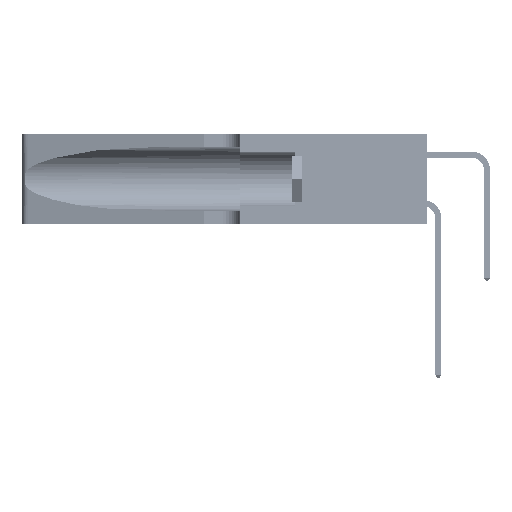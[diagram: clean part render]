
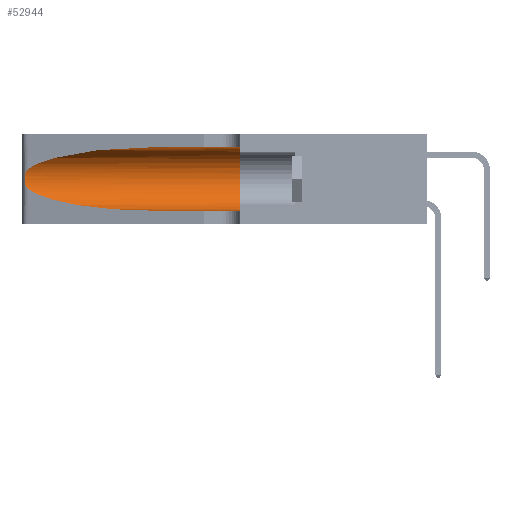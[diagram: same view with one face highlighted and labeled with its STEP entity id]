
A CAD part, left-side view. The second image highlights one B-rep face of the part: STEP entity #52944.
In plain terms, the highlighted cylindrical face has radius 3.308 mm (diameter 6.617 mm), a partial arc.
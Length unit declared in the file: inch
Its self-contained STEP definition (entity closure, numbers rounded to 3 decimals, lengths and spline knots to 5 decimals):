
#1289 = EDGE_CURVE ( 'NONE', #24550, #24707, #36671, .T. ) ;
#2194 = CARTESIAN_POINT ( 'NONE',  ( 0.26018, 1.23835, 0.19895 ) ) ;
#3975 = CARTESIAN_POINT ( 'NONE',  ( 0.18966, 0.96281, 0.31525 ) ) ;
#4296 = AXIS2_PLACEMENT_3D ( 'NONE', #30012, #25884, #5405 ) ;
#5024 = VERTEX_POINT ( 'NONE', #26585 ) ;
#5405 = DIRECTION ( 'NONE',  ( 0., 0., -1. ) ) ;
#6168 = CARTESIAN_POINT ( 'NONE',  ( 0.25555, 1.22994, 0.2215 ) ) ;
#6346 = CARTESIAN_POINT ( 'NONE',  ( 0.26075, 1.23896, 0.178 ) ) ;
#6778 = CARTESIAN_POINT ( 'NONE',  ( 0.1305, 1.61858, 0.31525 ) ) ;
#7345 = CARTESIAN_POINT ( 'NONE',  ( 0.18966, 0.96281, 0.05475 ) ) ;
#8405 = FACE_OUTER_BOUND ( 'NONE', #52028, .T. ) ;
#8641 = DIRECTION ( 'NONE',  ( 0., 1., 0. ) ) ;
#9437 = LINE ( 'NONE', #6778, #40942 ) ;
#9640 =( BOUNDED_CURVE ( )  B_SPLINE_CURVE ( 3, ( #27853, #52443, #7345, #36134 ),
 .UNSPECIFIED., .F., .T. ) 
 B_SPLINE_CURVE_WITH_KNOTS ( ( 4, 4 ),
 ( 3.44316, 4.71239 ),
 .UNSPECIFIED. ) 
 CURVE ( )  GEOMETRIC_REPRESENTATION_ITEM ( )  RATIONAL_B_SPLINE_CURVE ( ( 1., 0.87, 0.87, 1. ) ) 
 REPRESENTATION_ITEM ( '' )  );
#10225 = EDGE_CURVE ( 'NONE', #5024, #24550, #17521, .T. ) ;
#10495 = CARTESIAN_POINT ( 'NONE',  ( 0.25856, 1.23593, 0.16098 ) ) ;
#12281 = AXIS2_PLACEMENT_3D ( 'NONE', #33267, #8641, #37419 ) ;
#14595 = CARTESIAN_POINT ( 'NONE',  ( 0.25639, 1.23186, 0.15144 ) ) ;
#16179 = CIRCLE ( 'NONE', #12281, 0.13025 ) ;
#16218 = ORIENTED_EDGE ( 'NONE', *, *, #10225, .T. ) ;
#17521 =( BOUNDED_CURVE ( )  B_SPLINE_CURVE ( 3, ( #32737, #3975, #45147, #20523 ),
 .UNSPECIFIED., .F., .F. ) 
 B_SPLINE_CURVE_WITH_KNOTS ( ( 4, 4 ),
 ( 1.5708, 2.84003 ),
 .UNSPECIFIED. ) 
 CURVE ( )  GEOMETRIC_REPRESENTATION_ITEM ( )  RATIONAL_B_SPLINE_CURVE ( ( 1., 0.87, 0.87, 1. ) ) 
 REPRESENTATION_ITEM ( '' )  );
#17752 = CARTESIAN_POINT ( 'NONE',  ( 0.1305, 1.61858, 0.05475 ) ) ;
#18563 = CARTESIAN_POINT ( 'NONE',  ( 0.25639, 1.23184, 0.21858 ) ) ;
#18736 = CARTESIAN_POINT ( 'NONE',  ( 0.25487, 1.22718, 0.14631 ) ) ;
#20523 = CARTESIAN_POINT ( 'NONE',  ( 0.25487, 1.22718, 0.22369 ) ) ;
#20893 = CARTESIAN_POINT ( 'NONE',  ( 0.1305, 0.72297, 0.05475 ) ) ;
#22717 = CARTESIAN_POINT ( 'NONE',  ( 0.25487, 1.22718, 0.22369 ) ) ;
#24550 = VERTEX_POINT ( 'NONE', #39473 ) ;
#24707 = VERTEX_POINT ( 'NONE', #36575 ) ;
#24864 = VERTEX_POINT ( 'NONE', #20893 ) ;
#24978 = ORIENTED_EDGE ( 'NONE', *, *, #32246, .T. ) ;
#25884 = DIRECTION ( 'NONE',  ( 0., -1., 0. ) ) ;
#26585 = CARTESIAN_POINT ( 'NONE',  ( 0.1305, 0.72297, 0.31525 ) ) ;
#26829 = CARTESIAN_POINT ( 'NONE',  ( 0.25854, 1.2359, 0.20912 ) ) ;
#27078 = VECTOR ( 'NONE', #34307, 39.37008 ) ;
#27853 = CARTESIAN_POINT ( 'NONE',  ( 0.25487, 1.22718, 0.14631 ) ) ;
#27951 = CARTESIAN_POINT ( 'NONE',  ( 0.1305, 0.35, 0.05475 ) ) ;
#30012 = CARTESIAN_POINT ( 'NONE',  ( 0.1305, 1.61858, 0.185 ) ) ;
#30969 = CARTESIAN_POINT ( 'NONE',  ( 0.26075, 1.23896, 0.19203 ) ) ;
#31583 = ORIENTED_EDGE ( 'NONE', *, *, #1289, .T. ) ;
#32246 = EDGE_CURVE ( 'NONE', #24864, #35520, #40583, .T. ) ;
#32737 = CARTESIAN_POINT ( 'NONE',  ( 0.1305, 0.72297, 0.31525 ) ) ;
#33267 = CARTESIAN_POINT ( 'NONE',  ( 0.1305, 0.35, 0.185 ) ) ;
#34307 = DIRECTION ( 'NONE',  ( 0., -1., 0. ) ) ;
#35114 = CARTESIAN_POINT ( 'NONE',  ( 0.26017, 1.23833, 0.17102 ) ) ;
#35520 = VERTEX_POINT ( 'NONE', #27951 ) ;
#35771 = ORIENTED_EDGE ( 'NONE', *, *, #41002, .F. ) ;
#36134 = CARTESIAN_POINT ( 'NONE',  ( 0.1305, 0.72297, 0.05475 ) ) ;
#36146 = VERTEX_POINT ( 'NONE', #44068 ) ;
#36575 = CARTESIAN_POINT ( 'NONE',  ( 0.25487, 1.22718, 0.14631 ) ) ;
#36671 = B_SPLINE_CURVE_WITH_KNOTS ( 'NONE', 3,
 ( #22717, #6168, #18563, #51428, #26829, #2194, #30969, #6346, #35114, #10495, #39238, #14595, #43368, #18736 ),
 .UNSPECIFIED., .F., .F.,
 ( 4, 2, 2, 2, 2, 2, 4 ),
 ( 0., 0.00027, 0.00053, 0.00107, 0.0016, 0.00187, 0.00214 ),
 .UNSPECIFIED. ) ;
#37236 = ORIENTED_EDGE ( 'NONE', *, *, #38082, .T. ) ;
#37419 = DIRECTION ( 'NONE',  ( 0., 0., 1. ) ) ;
#38082 = EDGE_CURVE ( 'NONE', #24707, #24864, #9640, .T. ) ;
#39238 = CARTESIAN_POINT ( 'NONE',  ( 0.25789, 1.23486, 0.15765 ) ) ;
#39473 = CARTESIAN_POINT ( 'NONE',  ( 0.25487, 1.22718, 0.22369 ) ) ;
#39945 = CYLINDRICAL_SURFACE ( 'NONE', #4296, 0.13025 ) ;
#40583 = LINE ( 'NONE', #17752, #27078 ) ;
#40942 = VECTOR ( 'NONE', #47933, 39.37008 ) ;
#41002 = EDGE_CURVE ( 'NONE', #36146, #35520, #16179, .T. ) ;
#41895 = ORIENTED_EDGE ( 'NONE', *, *, #43864, .F. ) ;
#43368 = CARTESIAN_POINT ( 'NONE',  ( 0.25555, 1.22993, 0.14849 ) ) ;
#43864 = EDGE_CURVE ( 'NONE', #5024, #36146, #9437, .T. ) ;
#44068 = CARTESIAN_POINT ( 'NONE',  ( 0.1305, 0.35, 0.31525 ) ) ;
#45147 = CARTESIAN_POINT ( 'NONE',  ( 0.2373, 1.15595, 0.28018 ) ) ;
#47933 = DIRECTION ( 'NONE',  ( 0., -1., 0. ) ) ;
#51428 = CARTESIAN_POINT ( 'NONE',  ( 0.25787, 1.23484, 0.2124 ) ) ;
#52028 = EDGE_LOOP ( 'NONE', ( #16218, #31583, #37236, #24978, #35771, #41895 ) ) ;
#52443 = CARTESIAN_POINT ( 'NONE',  ( 0.2373, 1.15595, 0.08982 ) ) ;
#52944 = ADVANCED_FACE ( 'NONE', ( #8405 ), #39945, .F. ) ;
